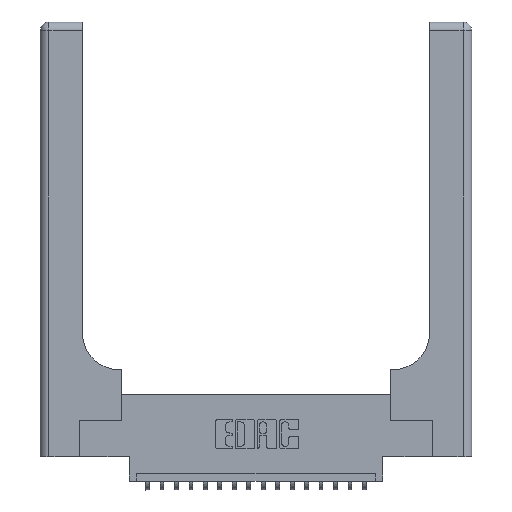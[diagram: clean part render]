
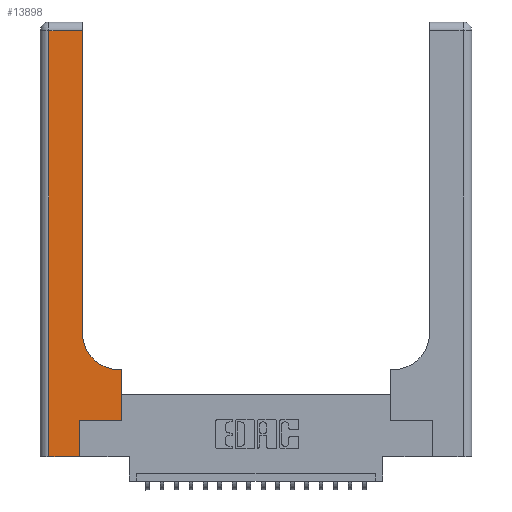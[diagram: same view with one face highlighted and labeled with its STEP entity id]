
A CAD part, top view. The second image highlights one B-rep face of the part: STEP entity #13898.
In plain terms, the highlighted planar face has unit normal (0, 0, 1).
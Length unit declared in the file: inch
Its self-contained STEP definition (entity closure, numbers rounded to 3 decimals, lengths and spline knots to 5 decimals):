
#231 = VECTOR ( 'NONE', #6847, 39.37008 ) ;
#473 = CARTESIAN_POINT ( 'NONE',  ( 0.2915, 2.94, 0.37 ) ) ;
#614 = CARTESIAN_POINT ( 'NONE',  ( 0.06, 3., 0.37 ) ) ;
#868 = VERTEX_POINT ( 'NONE', #18515 ) ;
#1241 = LINE ( 'NONE', #16861, #231 ) ;
#1296 = ORIENTED_EDGE ( 'NONE', *, *, #9150, .T. ) ;
#1561 = EDGE_CURVE ( 'NONE', #8633, #7390, #8445, .T. ) ;
#2115 = DIRECTION ( 'NONE',  ( 0., 1., 0. ) ) ;
#2668 = FACE_OUTER_BOUND ( 'NONE', #20122, .T. ) ;
#3247 = VECTOR ( 'NONE', #14038, 39.37008 ) ;
#3773 = EDGE_CURVE ( 'NONE', #12806, #15141, #11836, .T. ) ;
#3840 = ORIENTED_EDGE ( 'NONE', *, *, #7219, .T. ) ;
#3892 = DIRECTION ( 'NONE',  ( 0., 1., 0. ) ) ;
#4243 = ORIENTED_EDGE ( 'NONE', *, *, #4520, .T. ) ;
#4520 = EDGE_CURVE ( 'NONE', #15141, #18937, #17927, .T. ) ;
#5105 = VECTOR ( 'NONE', #11703, 39.37008 ) ;
#5111 = CARTESIAN_POINT ( 'NONE',  ( 0.5585, 0.25, 0.37 ) ) ;
#5189 = DIRECTION ( 'NONE',  ( -1., 0., 0. ) ) ;
#5245 = CARTESIAN_POINT ( 'NONE',  ( 0.5415, 0.6, 0.37 ) ) ;
#5457 = ORIENTED_EDGE ( 'NONE', *, *, #18354, .T. ) ;
#5639 = CARTESIAN_POINT ( 'NONE',  ( 0.2915, 0.6, 0.37 ) ) ;
#6421 = AXIS2_PLACEMENT_3D ( 'NONE', #18688, #13962, #15593 ) ;
#6538 = VERTEX_POINT ( 'NONE', #19699 ) ;
#6847 = DIRECTION ( 'NONE',  ( 0., 1., 0. ) ) ;
#7161 = ORIENTED_EDGE ( 'NONE', *, *, #1561, .T. ) ;
#7219 = EDGE_CURVE ( 'NONE', #14625, #12806, #7644, .T. ) ;
#7390 = VERTEX_POINT ( 'NONE', #18236 ) ;
#7644 = LINE ( 'NONE', #8283, #16053 ) ;
#8249 = CARTESIAN_POINT ( 'NONE',  ( 0.269, 0.25, 0.37 ) ) ;
#8283 = CARTESIAN_POINT ( 'NONE',  ( 0., 2.94, 0.37 ) ) ;
#8445 = CIRCLE ( 'NONE', #6421, 0.25 ) ;
#8633 = VERTEX_POINT ( 'NONE', #5245 ) ;
#8658 = VECTOR ( 'NONE', #10649, 39.37008 ) ;
#8990 = CARTESIAN_POINT ( 'NONE',  ( 0., 3., 0.37 ) ) ;
#9150 = EDGE_CURVE ( 'NONE', #18937, #6538, #17283, .T. ) ;
#9480 = EDGE_CURVE ( 'NONE', #11817, #8633, #13695, .T. ) ;
#10521 = PLANE ( 'NONE',  #12867 ) ;
#10649 = DIRECTION ( 'NONE',  ( -1., 0., 0. ) ) ;
#11703 = DIRECTION ( 'NONE',  ( 1., 0., 0. ) ) ;
#11770 = CARTESIAN_POINT ( 'NONE',  ( 0.269, 0., 0.37 ) ) ;
#11817 = VERTEX_POINT ( 'NONE', #13380 ) ;
#11836 = LINE ( 'NONE', #614, #3247 ) ;
#11918 = CARTESIAN_POINT ( 'NONE',  ( 0.06, 2.94, 0.37 ) ) ;
#12622 = ORIENTED_EDGE ( 'NONE', *, *, #3773, .T. ) ;
#12806 = VERTEX_POINT ( 'NONE', #11918 ) ;
#12867 = AXIS2_PLACEMENT_3D ( 'NONE', #8990, #18726, #18797 ) ;
#13380 = CARTESIAN_POINT ( 'NONE',  ( 0.5585, 0.6, 0.37 ) ) ;
#13695 = LINE ( 'NONE', #5639, #8658 ) ;
#13898 = ADVANCED_FACE ( 'NONE', ( #2668 ), #10521, .F. ) ;
#13962 = DIRECTION ( 'NONE',  ( 0., 0., -1. ) ) ;
#14038 = DIRECTION ( 'NONE',  ( 0., -1., 0. ) ) ;
#14471 = CARTESIAN_POINT ( 'NONE',  ( 0.269, 0., 0.37 ) ) ;
#14625 = VERTEX_POINT ( 'NONE', #473 ) ;
#14759 = VECTOR ( 'NONE', #3892, 39.37008 ) ;
#14888 = ORIENTED_EDGE ( 'NONE', *, *, #14911, .T. ) ;
#14911 = EDGE_CURVE ( 'NONE', #6538, #868, #20826, .T. ) ;
#15141 = VERTEX_POINT ( 'NONE', #19435 ) ;
#15399 = DIRECTION ( 'NONE',  ( 1., 0., 0. ) ) ;
#15593 = DIRECTION ( 'NONE',  ( 1., 0., 0. ) ) ;
#16053 = VECTOR ( 'NONE', #5189, 39.37008 ) ;
#16827 = ORIENTED_EDGE ( 'NONE', *, *, #9480, .T. ) ;
#16861 = CARTESIAN_POINT ( 'NONE',  ( 0.2915, 3., 0.37 ) ) ;
#16925 = ORIENTED_EDGE ( 'NONE', *, *, #17198, .T. ) ;
#17021 = CARTESIAN_POINT ( 'NONE',  ( 0., 0., 0.37 ) ) ;
#17198 = EDGE_CURVE ( 'NONE', #7390, #14625, #1241, .T. ) ;
#17283 = LINE ( 'NONE', #11770, #14759 ) ;
#17649 = LINE ( 'NONE', #5111, #20668 ) ;
#17927 = LINE ( 'NONE', #17021, #20697 ) ;
#18236 = CARTESIAN_POINT ( 'NONE',  ( 0.2915, 0.85, 0.37 ) ) ;
#18354 = EDGE_CURVE ( 'NONE', #868, #11817, #17649, .T. ) ;
#18515 = CARTESIAN_POINT ( 'NONE',  ( 0.5585, 0.25, 0.37 ) ) ;
#18688 = CARTESIAN_POINT ( 'NONE',  ( 0.5415, 0.85, 0.37 ) ) ;
#18726 = DIRECTION ( 'NONE',  ( 0., 0., -1. ) ) ;
#18797 = DIRECTION ( 'NONE',  ( -1., 0., 0. ) ) ;
#18937 = VERTEX_POINT ( 'NONE', #14471 ) ;
#19435 = CARTESIAN_POINT ( 'NONE',  ( 0.06, 0., 0.37 ) ) ;
#19699 = CARTESIAN_POINT ( 'NONE',  ( 0.269, 0.25, 0.37 ) ) ;
#20122 = EDGE_LOOP ( 'NONE', ( #16925, #3840, #12622, #4243, #1296, #14888, #5457, #16827, #7161 ) ) ;
#20668 = VECTOR ( 'NONE', #2115, 39.37008 ) ;
#20697 = VECTOR ( 'NONE', #15399, 39.37008 ) ;
#20826 = LINE ( 'NONE', #8249, #5105 ) ;
